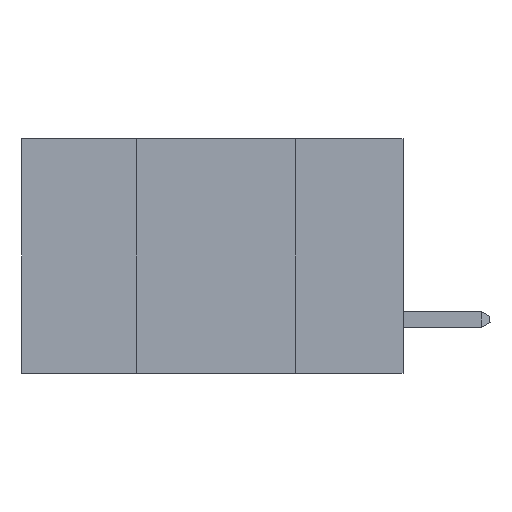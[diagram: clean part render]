
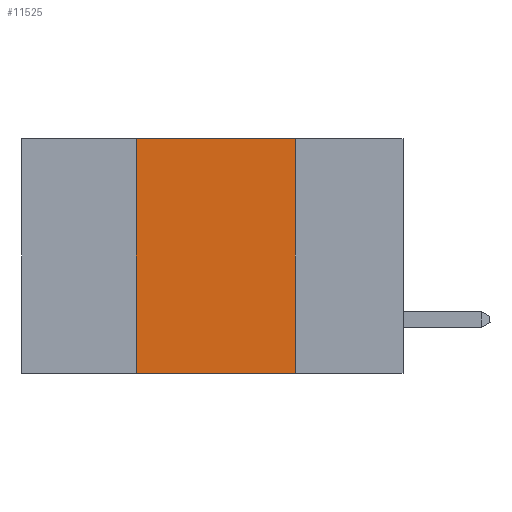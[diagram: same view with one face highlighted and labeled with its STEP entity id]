
A CAD part, left-side view. The second image highlights one B-rep face of the part: STEP entity #11525.
In plain terms, the highlighted planar face has unit normal (-1, 0, 0).
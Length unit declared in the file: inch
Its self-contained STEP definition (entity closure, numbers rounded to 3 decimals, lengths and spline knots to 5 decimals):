
#437 = CARTESIAN_POINT ( 'NONE',  ( 0., 0.17, 0. ) ) ;
#1809 = EDGE_CURVE ( 'NONE', #29642, #21489, #31176, .T. ) ;
#2239 = PLANE ( 'NONE',  #37879 ) ;
#2554 = FACE_OUTER_BOUND ( 'NONE', #11304, .T. ) ;
#6477 = CARTESIAN_POINT ( 'NONE',  ( 0., 0.6, -0.37 ) ) ;
#8369 = EDGE_CURVE ( 'NONE', #29642, #43250, #18427, .T. ) ;
#9173 = CARTESIAN_POINT ( 'NONE',  ( 0., 0.17, 0. ) ) ;
#11304 = EDGE_LOOP ( 'NONE', ( #25415, #28549, #32366, #44585 ) ) ;
#11399 = LINE ( 'NONE', #437, #45129 ) ;
#11525 = ADVANCED_FACE ( 'NONE', ( #2554 ), #2239, .F. ) ;
#11853 = VECTOR ( 'NONE', #44332, 39.37008 ) ;
#18427 = LINE ( 'NONE', #30322, #24689 ) ;
#19911 = DIRECTION ( 'NONE',  ( 1., 0., 0. ) ) ;
#21420 = LINE ( 'NONE', #40566, #11853 ) ;
#21489 = VERTEX_POINT ( 'NONE', #44383 ) ;
#21968 = DIRECTION ( 'NONE',  ( 0., -1., 0. ) ) ;
#22718 = EDGE_CURVE ( 'NONE', #43250, #22789, #21420, .T. ) ;
#22789 = VERTEX_POINT ( 'NONE', #9173 ) ;
#24689 = VECTOR ( 'NONE', #44920, 39.37008 ) ;
#25415 = ORIENTED_EDGE ( 'NONE', *, *, #31318, .F. ) ;
#28549 = ORIENTED_EDGE ( 'NONE', *, *, #22718, .F. ) ;
#28893 = DIRECTION ( 'NONE',  ( 0., 0., -1. ) ) ;
#29642 = VERTEX_POINT ( 'NONE', #40209 ) ;
#30322 = CARTESIAN_POINT ( 'NONE',  ( 0., 0.42, 0. ) ) ;
#31176 = LINE ( 'NONE', #6477, #37969 ) ;
#31318 = EDGE_CURVE ( 'NONE', #22789, #21489, #11399, .T. ) ;
#32366 = ORIENTED_EDGE ( 'NONE', *, *, #8369, .F. ) ;
#34616 = CARTESIAN_POINT ( 'NONE',  ( 0., 0.6, 0. ) ) ;
#37752 = DIRECTION ( 'NONE',  ( 0., 0., -1. ) ) ;
#37879 = AXIS2_PLACEMENT_3D ( 'NONE', #34616, #19911, #37752 ) ;
#37969 = VECTOR ( 'NONE', #21968, 39.37008 ) ;
#39964 = CARTESIAN_POINT ( 'NONE',  ( 0., 0.42, 0. ) ) ;
#40209 = CARTESIAN_POINT ( 'NONE',  ( 0., 0.42, -0.37 ) ) ;
#40566 = CARTESIAN_POINT ( 'NONE',  ( 0., 0.6, 0. ) ) ;
#43250 = VERTEX_POINT ( 'NONE', #39964 ) ;
#44332 = DIRECTION ( 'NONE',  ( 0., -1., 0. ) ) ;
#44383 = CARTESIAN_POINT ( 'NONE',  ( 0., 0.17, -0.37 ) ) ;
#44585 = ORIENTED_EDGE ( 'NONE', *, *, #1809, .T. ) ;
#44920 = DIRECTION ( 'NONE',  ( 0., 0., 1. ) ) ;
#45129 = VECTOR ( 'NONE', #28893, 39.37008 ) ;
